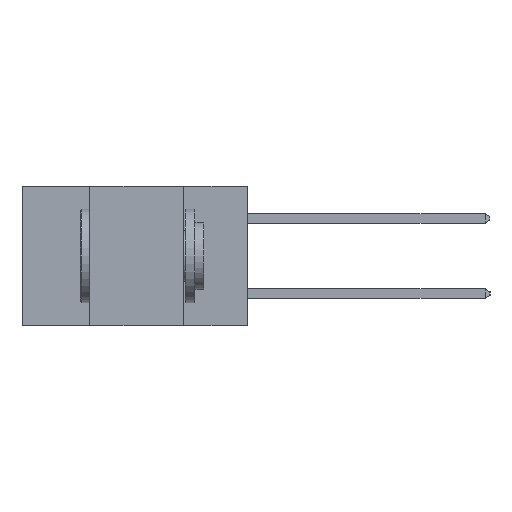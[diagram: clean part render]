
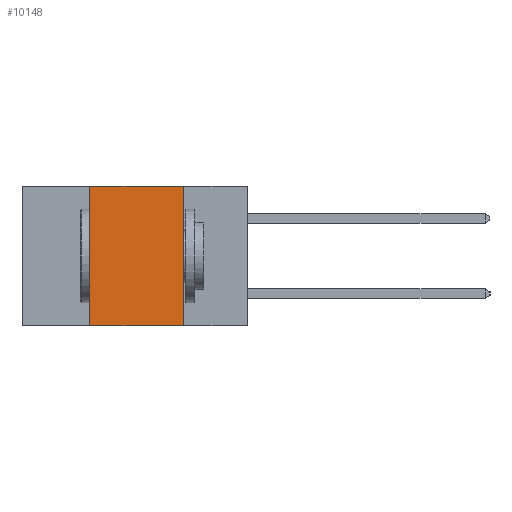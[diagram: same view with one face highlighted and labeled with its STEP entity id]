
A CAD part, left-side view. The second image highlights one B-rep face of the part: STEP entity #10148.
In plain terms, the highlighted planar face has unit normal (-1, 0, 0).
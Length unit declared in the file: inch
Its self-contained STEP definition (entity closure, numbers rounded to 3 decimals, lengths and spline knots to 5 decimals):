
#39 = FACE_OUTER_BOUND ( 'NONE', #3392, .T. ) ;
#863 = CARTESIAN_POINT ( 'NONE',  ( 0., 0.42, 0. ) ) ;
#1706 = EDGE_CURVE ( 'NONE', #10113, #6809, #8074, .T. ) ;
#2017 = VERTEX_POINT ( 'NONE', #3650 ) ;
#2360 = DIRECTION ( 'NONE',  ( 0., -1., 0. ) ) ;
#2464 = VECTOR ( 'NONE', #9143, 39.37008 ) ;
#2590 = CARTESIAN_POINT ( 'NONE',  ( 0., 0.6, 0. ) ) ;
#3244 = LINE ( 'NONE', #2590, #11269 ) ;
#3392 = EDGE_LOOP ( 'NONE', ( #5203, #12319, #5859, #7698 ) ) ;
#3465 = VECTOR ( 'NONE', #8943, 39.37008 ) ;
#3650 = CARTESIAN_POINT ( 'NONE',  ( 0., 0.17, -0.37 ) ) ;
#3774 = LINE ( 'NONE', #13168, #3465 ) ;
#4171 = VERTEX_POINT ( 'NONE', #5120 ) ;
#4579 = EDGE_CURVE ( 'NONE', #10113, #2017, #11754, .T. ) ;
#5120 = CARTESIAN_POINT ( 'NONE',  ( 0., 0.17, 0. ) ) ;
#5203 = ORIENTED_EDGE ( 'NONE', *, *, #9878, .F. ) ;
#5859 = ORIENTED_EDGE ( 'NONE', *, *, #1706, .F. ) ;
#6232 = EDGE_CURVE ( 'NONE', #6809, #4171, #3244, .T. ) ;
#6809 = VERTEX_POINT ( 'NONE', #863 ) ;
#6823 = AXIS2_PLACEMENT_3D ( 'NONE', #11589, #11504, #11492 ) ;
#7347 = CARTESIAN_POINT ( 'NONE',  ( 0., 0.42, -0.37 ) ) ;
#7698 = ORIENTED_EDGE ( 'NONE', *, *, #4579, .T. ) ;
#8074 = LINE ( 'NONE', #7347, #2464 ) ;
#8943 = DIRECTION ( 'NONE',  ( 0., 0., -1. ) ) ;
#9043 = VECTOR ( 'NONE', #13003, 39.37008 ) ;
#9143 = DIRECTION ( 'NONE',  ( 0., 0., 1. ) ) ;
#9878 = EDGE_CURVE ( 'NONE', #4171, #2017, #3774, .T. ) ;
#10113 = VERTEX_POINT ( 'NONE', #11829 ) ;
#10148 = ADVANCED_FACE ( 'NONE', ( #39 ), #11519, .F. ) ;
#11269 = VECTOR ( 'NONE', #2360, 39.37008 ) ;
#11492 = DIRECTION ( 'NONE',  ( 0., 0., -1. ) ) ;
#11504 = DIRECTION ( 'NONE',  ( 1., 0., 0. ) ) ;
#11519 = PLANE ( 'NONE',  #6823 ) ;
#11589 = CARTESIAN_POINT ( 'NONE',  ( 0., 0.6, 0. ) ) ;
#11754 = LINE ( 'NONE', #13081, #9043 ) ;
#11829 = CARTESIAN_POINT ( 'NONE',  ( 0., 0.42, -0.37 ) ) ;
#12319 = ORIENTED_EDGE ( 'NONE', *, *, #6232, .F. ) ;
#13003 = DIRECTION ( 'NONE',  ( 0., -1., 0. ) ) ;
#13081 = CARTESIAN_POINT ( 'NONE',  ( 0., 0.6, -0.37 ) ) ;
#13168 = CARTESIAN_POINT ( 'NONE',  ( 0., 0.17, -0.37 ) ) ;
